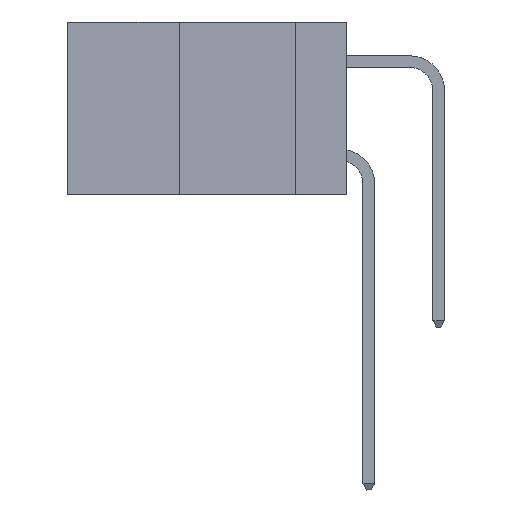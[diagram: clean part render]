
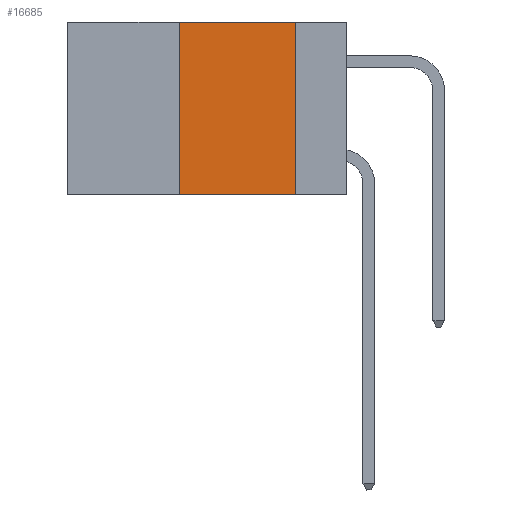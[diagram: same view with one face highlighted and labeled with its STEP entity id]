
A CAD part, left-side view. The second image highlights one B-rep face of the part: STEP entity #16685.
In plain terms, the highlighted planar face has unit normal (-1, 0, 0).
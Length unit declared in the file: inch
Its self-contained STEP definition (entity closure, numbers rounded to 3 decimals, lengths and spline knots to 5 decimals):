
#18 = CARTESIAN_POINT ( 'NONE',  ( 0., 0.36, -0.37 ) ) ;
#221 = CARTESIAN_POINT ( 'NONE',  ( 0., 0.11, 0. ) ) ;
#2069 = CARTESIAN_POINT ( 'NONE',  ( 0., 0.6, -0.37 ) ) ;
#2736 = DIRECTION ( 'NONE',  ( 0., 0., 1. ) ) ;
#2777 = VERTEX_POINT ( 'NONE', #10227 ) ;
#3061 = VERTEX_POINT ( 'NONE', #221 ) ;
#3063 = DIRECTION ( 'NONE',  ( 1., 0., 0. ) ) ;
#4077 = CARTESIAN_POINT ( 'NONE',  ( 0., 0.36, 0. ) ) ;
#4217 = VECTOR ( 'NONE', #11617, 39.37008 ) ;
#5004 = CARTESIAN_POINT ( 'NONE',  ( 0., 0.11, 0. ) ) ;
#5581 = VERTEX_POINT ( 'NONE', #18 ) ;
#6335 = LINE ( 'NONE', #5004, #4217 ) ;
#6968 = VERTEX_POINT ( 'NONE', #9925 ) ;
#7338 = PLANE ( 'NONE',  #7761 ) ;
#7612 = ORIENTED_EDGE ( 'NONE', *, *, #15306, .F. ) ;
#7761 = AXIS2_PLACEMENT_3D ( 'NONE', #16804, #3063, #15377 ) ;
#8686 = CARTESIAN_POINT ( 'NONE',  ( 0., 0.6, 0. ) ) ;
#8767 = FACE_OUTER_BOUND ( 'NONE', #17112, .T. ) ;
#9729 = ORIENTED_EDGE ( 'NONE', *, *, #16623, .F. ) ;
#9925 = CARTESIAN_POINT ( 'NONE',  ( 0., 0.36, 0. ) ) ;
#10117 = LINE ( 'NONE', #8686, #15163 ) ;
#10186 = DIRECTION ( 'NONE',  ( 0., -1., 0. ) ) ;
#10227 = CARTESIAN_POINT ( 'NONE',  ( 0., 0.11, -0.37 ) ) ;
#10786 = VECTOR ( 'NONE', #10186, 39.37008 ) ;
#11532 = LINE ( 'NONE', #2069, #10786 ) ;
#11617 = DIRECTION ( 'NONE',  ( 0., 0., -1. ) ) ;
#12646 = ORIENTED_EDGE ( 'NONE', *, *, #14124, .F. ) ;
#12912 = EDGE_CURVE ( 'NONE', #5581, #2777, #11532, .T. ) ;
#13890 = ORIENTED_EDGE ( 'NONE', *, *, #12912, .T. ) ;
#13976 = LINE ( 'NONE', #4077, #16894 ) ;
#14124 = EDGE_CURVE ( 'NONE', #3061, #2777, #6335, .T. ) ;
#15163 = VECTOR ( 'NONE', #15293, 39.37008 ) ;
#15293 = DIRECTION ( 'NONE',  ( 0., -1., 0. ) ) ;
#15306 = EDGE_CURVE ( 'NONE', #5581, #6968, #13976, .T. ) ;
#15377 = DIRECTION ( 'NONE',  ( 0., 0., -1. ) ) ;
#16623 = EDGE_CURVE ( 'NONE', #6968, #3061, #10117, .T. ) ;
#16685 = ADVANCED_FACE ( 'NONE', ( #8767 ), #7338, .F. ) ;
#16804 = CARTESIAN_POINT ( 'NONE',  ( 0., 0.6, 0. ) ) ;
#16894 = VECTOR ( 'NONE', #2736, 39.37008 ) ;
#17112 = EDGE_LOOP ( 'NONE', ( #12646, #9729, #7612, #13890 ) ) ;
